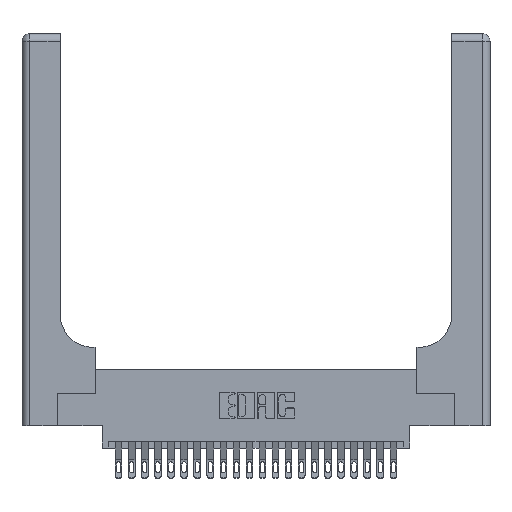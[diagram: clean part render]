
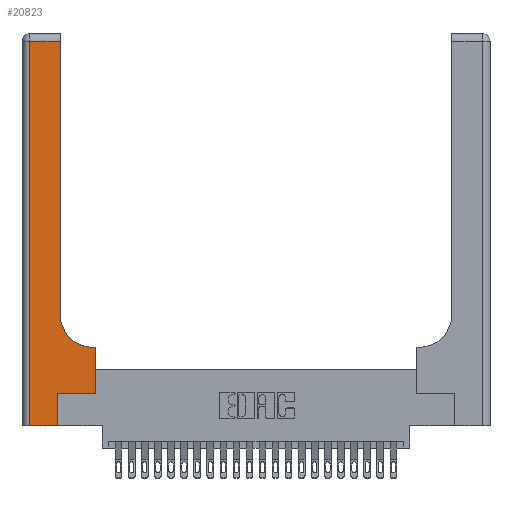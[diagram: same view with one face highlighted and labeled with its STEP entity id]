
A CAD part, top view. The second image highlights one B-rep face of the part: STEP entity #20823.
In plain terms, the highlighted planar face has unit normal (0, 0, 1).
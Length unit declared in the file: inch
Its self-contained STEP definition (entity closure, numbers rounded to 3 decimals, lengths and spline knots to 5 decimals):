
#145 = CARTESIAN_POINT ( 'NONE',  ( 0.269, 0., 0.37 ) ) ;
#770 = ORIENTED_EDGE ( 'NONE', *, *, #7813, .T. ) ;
#1166 = ORIENTED_EDGE ( 'NONE', *, *, #9532, .T. ) ;
#1530 = CARTESIAN_POINT ( 'NONE',  ( 0.5585, 0.6, 0.37 ) ) ;
#2443 = CARTESIAN_POINT ( 'NONE',  ( 0.06, 2.94, 0.37 ) ) ;
#2445 = VECTOR ( 'NONE', #6327, 39.37008 ) ;
#4467 = CARTESIAN_POINT ( 'NONE',  ( 0.5415, 0.6, 0.37 ) ) ;
#4968 = CARTESIAN_POINT ( 'NONE',  ( 0.5415, 0.85, 0.37 ) ) ;
#5515 = CIRCLE ( 'NONE', #16412, 0.25 ) ;
#5743 = LINE ( 'NONE', #19300, #11723 ) ;
#6327 = DIRECTION ( 'NONE',  ( 0., 1., 0. ) ) ;
#6331 = VERTEX_POINT ( 'NONE', #1530 ) ;
#6534 = ORIENTED_EDGE ( 'NONE', *, *, #13696, .T. ) ;
#6916 = VERTEX_POINT ( 'NONE', #19006 ) ;
#6921 = CARTESIAN_POINT ( 'NONE',  ( 0.2915, 3., 0.37 ) ) ;
#6972 = VECTOR ( 'NONE', #14802, 39.37008 ) ;
#7009 = DIRECTION ( 'NONE',  ( 1., 0., 0. ) ) ;
#7331 = EDGE_CURVE ( 'NONE', #17963, #23117, #11541, .T. ) ;
#7813 = EDGE_CURVE ( 'NONE', #23727, #8659, #5515, .T. ) ;
#7892 = CARTESIAN_POINT ( 'NONE',  ( 0.06, 0., 0.37 ) ) ;
#8005 = DIRECTION ( 'NONE',  ( -1., 0., 0. ) ) ;
#8382 = EDGE_CURVE ( 'NONE', #8862, #6331, #13601, .T. ) ;
#8659 = VERTEX_POINT ( 'NONE', #9283 ) ;
#8862 = VERTEX_POINT ( 'NONE', #23348 ) ;
#9283 = CARTESIAN_POINT ( 'NONE',  ( 0.2915, 0.85, 0.37 ) ) ;
#9532 = EDGE_CURVE ( 'NONE', #6916, #24680, #10360, .T. ) ;
#10203 = CARTESIAN_POINT ( 'NONE',  ( 0., 2.94, 0.37 ) ) ;
#10360 = LINE ( 'NONE', #10203, #20014 ) ;
#11541 = LINE ( 'NONE', #18648, #21174 ) ;
#11723 = VECTOR ( 'NONE', #15453, 39.37008 ) ;
#11873 = ORIENTED_EDGE ( 'NONE', *, *, #7331, .T. ) ;
#12153 = DIRECTION ( 'NONE',  ( -1., 0., 0. ) ) ;
#12543 = CARTESIAN_POINT ( 'NONE',  ( 0.5585, 0.25, 0.37 ) ) ;
#12619 = EDGE_LOOP ( 'NONE', ( #20687, #1166, #20019, #11873, #20933, #18523, #12793, #6534, #770 ) ) ;
#12793 = ORIENTED_EDGE ( 'NONE', *, *, #8382, .T. ) ;
#12927 = DIRECTION ( 'NONE',  ( 1., 0., 0. ) ) ;
#13601 = LINE ( 'NONE', #12543, #23884 ) ;
#13680 = DIRECTION ( 'NONE',  ( 1., 0., 0. ) ) ;
#13696 = EDGE_CURVE ( 'NONE', #6331, #23727, #5743, .T. ) ;
#13890 = CARTESIAN_POINT ( 'NONE',  ( 0., 3., 0.37 ) ) ;
#14802 = DIRECTION ( 'NONE',  ( 0., 1., 0. ) ) ;
#14989 = CARTESIAN_POINT ( 'NONE',  ( 0.06, 3., 0.37 ) ) ;
#15453 = DIRECTION ( 'NONE',  ( -1., 0., 0. ) ) ;
#15973 = VERTEX_POINT ( 'NONE', #16435 ) ;
#16412 = AXIS2_PLACEMENT_3D ( 'NONE', #4968, #18722, #7009 ) ;
#16435 = CARTESIAN_POINT ( 'NONE',  ( 0.269, 0.25, 0.37 ) ) ;
#16441 = DIRECTION ( 'NONE',  ( 0., 1., 0. ) ) ;
#16505 = VECTOR ( 'NONE', #13680, 39.37008 ) ;
#17443 = VECTOR ( 'NONE', #22739, 39.37008 ) ;
#17963 = VERTEX_POINT ( 'NONE', #7892 ) ;
#18523 = ORIENTED_EDGE ( 'NONE', *, *, #20070, .T. ) ;
#18648 = CARTESIAN_POINT ( 'NONE',  ( 0., 0., 0.37 ) ) ;
#18722 = DIRECTION ( 'NONE',  ( 0., 0., -1. ) ) ;
#19006 = CARTESIAN_POINT ( 'NONE',  ( 0.2915, 2.94, 0.37 ) ) ;
#19300 = CARTESIAN_POINT ( 'NONE',  ( 0.2915, 0.6, 0.37 ) ) ;
#19336 = EDGE_CURVE ( 'NONE', #24680, #17963, #22584, .T. ) ;
#19658 = DIRECTION ( 'NONE',  ( 0., 0., -1. ) ) ;
#19796 = EDGE_CURVE ( 'NONE', #8659, #6916, #22558, .T. ) ;
#20014 = VECTOR ( 'NONE', #12153, 39.37008 ) ;
#20019 = ORIENTED_EDGE ( 'NONE', *, *, #19336, .T. ) ;
#20070 = EDGE_CURVE ( 'NONE', #15973, #8862, #21008, .T. ) ;
#20670 = FACE_OUTER_BOUND ( 'NONE', #12619, .T. ) ;
#20687 = ORIENTED_EDGE ( 'NONE', *, *, #19796, .T. ) ;
#20823 = ADVANCED_FACE ( 'NONE', ( #20670 ), #23517, .F. ) ;
#20931 = EDGE_CURVE ( 'NONE', #23117, #15973, #23404, .T. ) ;
#20933 = ORIENTED_EDGE ( 'NONE', *, *, #20931, .T. ) ;
#21008 = LINE ( 'NONE', #25260, #16505 ) ;
#21174 = VECTOR ( 'NONE', #12927, 39.37008 ) ;
#22272 = AXIS2_PLACEMENT_3D ( 'NONE', #13890, #19658, #8005 ) ;
#22558 = LINE ( 'NONE', #6921, #6972 ) ;
#22584 = LINE ( 'NONE', #14989, #17443 ) ;
#22739 = DIRECTION ( 'NONE',  ( 0., -1., 0. ) ) ;
#23117 = VERTEX_POINT ( 'NONE', #23637 ) ;
#23348 = CARTESIAN_POINT ( 'NONE',  ( 0.5585, 0.25, 0.37 ) ) ;
#23404 = LINE ( 'NONE', #145, #2445 ) ;
#23517 = PLANE ( 'NONE',  #22272 ) ;
#23637 = CARTESIAN_POINT ( 'NONE',  ( 0.269, 0., 0.37 ) ) ;
#23727 = VERTEX_POINT ( 'NONE', #4467 ) ;
#23884 = VECTOR ( 'NONE', #16441, 39.37008 ) ;
#24680 = VERTEX_POINT ( 'NONE', #2443 ) ;
#25260 = CARTESIAN_POINT ( 'NONE',  ( 0.269, 0.25, 0.37 ) ) ;
